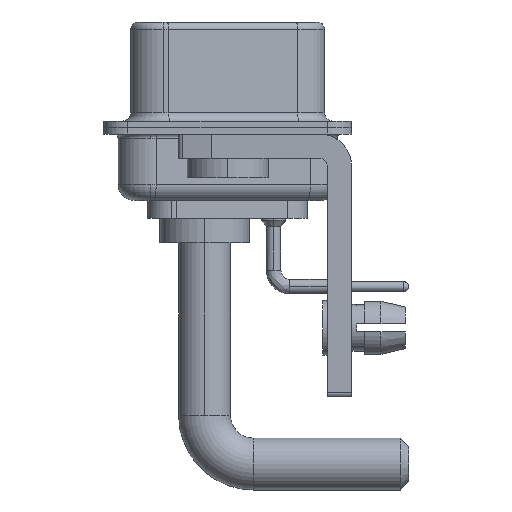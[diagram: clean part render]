
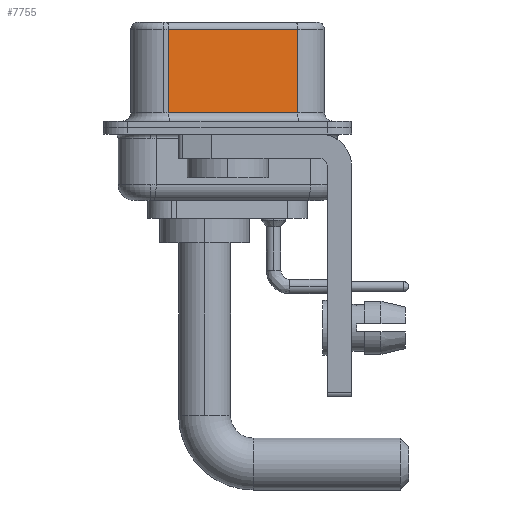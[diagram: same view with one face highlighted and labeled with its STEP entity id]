
A CAD part, left-side view. The second image highlights one B-rep face of the part: STEP entity #7755.
In plain terms, the highlighted planar face has unit normal (-0.985, -0.174, 0).
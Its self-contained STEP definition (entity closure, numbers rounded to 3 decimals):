
#263 = VERTEX_POINT ( 'NONE', #13987 ) ;
#1545 = CARTESIAN_POINT ( 'NONE',  ( 5.132, -4.322, 6.52 ) ) ;
#1567 = LINE ( 'NONE', #9725, #20144 ) ;
#1606 = EDGE_LOOP ( 'NONE', ( #18035, #2766, #17766, #24927 ) ) ;
#2766 = ORIENTED_EDGE ( 'NONE', *, *, #25231, .T. ) ;
#4559 = LINE ( 'NONE', #18982, #6442 ) ;
#4870 = LINE ( 'NONE', #19429, #8016 ) ;
#5373 = VERTEX_POINT ( 'NONE', #18453 ) ;
#6083 = PLANE ( 'NONE',  #13394 ) ;
#6183 = CARTESIAN_POINT ( 'NONE',  ( 5.132, -4.322, 6.02 ) ) ;
#6207 = EDGE_CURVE ( 'NONE', #12868, #5373, #1567, .T. ) ;
#6442 = VECTOR ( 'NONE', #12983, 1000. ) ;
#7755 = ADVANCED_FACE ( 'NONE', ( #15966 ), #6083, .F. ) ;
#7789 = VERTEX_POINT ( 'NONE', #22818 ) ;
#8016 = VECTOR ( 'NONE', #19162, 1000. ) ;
#8477 = CARTESIAN_POINT ( 'NONE',  ( 3.73, 3.628, 6.52 ) ) ;
#9725 = CARTESIAN_POINT ( 'NONE',  ( 5.132, -4.322, 6.52 ) ) ;
#11969 = DIRECTION ( 'NONE',  ( 0.985, 0.174, 0. ) ) ;
#12868 = VERTEX_POINT ( 'NONE', #6183 ) ;
#12879 = LINE ( 'NONE', #8477, #24678 ) ;
#12983 = DIRECTION ( 'NONE',  ( -0.174, 0.985, 0. ) ) ;
#13394 = AXIS2_PLACEMENT_3D ( 'NONE', #1545, #11969, #20108 ) ;
#13675 = EDGE_CURVE ( 'NONE', #7789, #5373, #4870, .T. ) ;
#13987 = CARTESIAN_POINT ( 'NONE',  ( 3.73, 3.628, 6.02 ) ) ;
#15966 = FACE_OUTER_BOUND ( 'NONE', #1606, .T. ) ;
#17766 = ORIENTED_EDGE ( 'NONE', *, *, #20462, .T. ) ;
#17872 = DIRECTION ( 'NONE',  ( 0., 0., -1. ) ) ;
#18035 = ORIENTED_EDGE ( 'NONE', *, *, #6207, .F. ) ;
#18453 = CARTESIAN_POINT ( 'NONE',  ( 5.132, -4.322, 0.9 ) ) ;
#18756 = DIRECTION ( 'NONE',  ( 0., 0., -1. ) ) ;
#18982 = CARTESIAN_POINT ( 'NONE',  ( 5.132, -4.322, 6.02 ) ) ;
#19162 = DIRECTION ( 'NONE',  ( 0.174, -0.985, 0. ) ) ;
#19429 = CARTESIAN_POINT ( 'NONE',  ( 5.132, -4.322, 0.9 ) ) ;
#20108 = DIRECTION ( 'NONE',  ( -0.174, 0.985, 0. ) ) ;
#20144 = VECTOR ( 'NONE', #17872, 1000. ) ;
#20462 = EDGE_CURVE ( 'NONE', #263, #7789, #12879, .T. ) ;
#22818 = CARTESIAN_POINT ( 'NONE',  ( 3.73, 3.628, 0.9 ) ) ;
#24678 = VECTOR ( 'NONE', #18756, 1000. ) ;
#24927 = ORIENTED_EDGE ( 'NONE', *, *, #13675, .T. ) ;
#25231 = EDGE_CURVE ( 'NONE', #12868, #263, #4559, .T. ) ;
